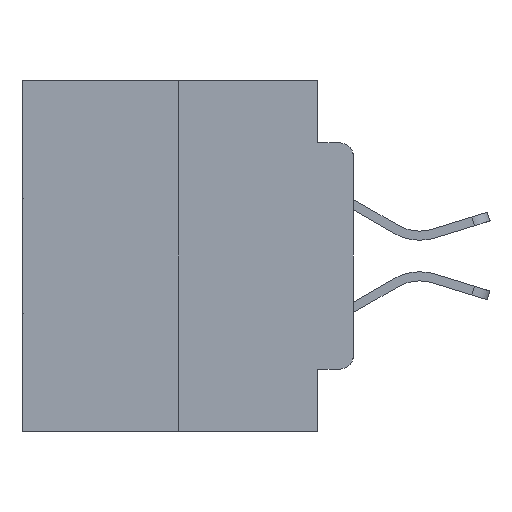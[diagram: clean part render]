
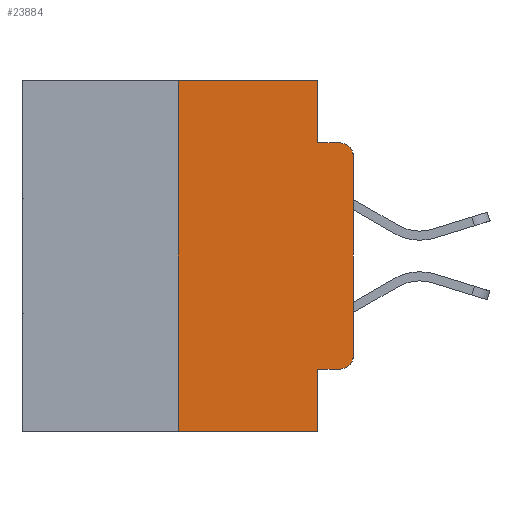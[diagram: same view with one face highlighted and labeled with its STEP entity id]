
A CAD part, left-side view. The second image highlights one B-rep face of the part: STEP entity #23884.
In plain terms, the highlighted planar face has unit normal (-1, 0, 0).
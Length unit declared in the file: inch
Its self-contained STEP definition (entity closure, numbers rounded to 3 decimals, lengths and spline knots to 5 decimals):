
#173 = CARTESIAN_POINT ( 'NONE',  ( 0., 0.051, -0.4115 ) ) ;
#317 = AXIS2_PLACEMENT_3D ( 'NONE', #12947, #27071, #15091 ) ;
#644 = CARTESIAN_POINT ( 'NONE',  ( 0., 0.051, 0. ) ) ;
#1097 = ORIENTED_EDGE ( 'NONE', *, *, #15920, .T. ) ;
#1179 = CARTESIAN_POINT ( 'NONE',  ( 0., 0.051, -0.0885 ) ) ;
#1443 = CARTESIAN_POINT ( 'NONE',  ( 0., 0., -0.1085 ) ) ;
#1916 = CARTESIAN_POINT ( 'NONE',  ( 0., 0., -0.3915 ) ) ;
#1993 = VERTEX_POINT ( 'NONE', #1443 ) ;
#2488 = DIRECTION ( 'NONE',  ( 0., -1., 0. ) ) ;
#2595 = EDGE_CURVE ( 'NONE', #9877, #24807, #21165, .T. ) ;
#2818 = DIRECTION ( 'NONE',  ( 0., 0., -1. ) ) ;
#2937 = LINE ( 'NONE', #7211, #19235 ) ;
#3059 = CARTESIAN_POINT ( 'NONE',  ( 0., 0.02, -0.0885 ) ) ;
#3100 = VERTEX_POINT ( 'NONE', #1916 ) ;
#3442 = VERTEX_POINT ( 'NONE', #3059 ) ;
#3633 = VECTOR ( 'NONE', #2488, 39.37008 ) ;
#3648 = VECTOR ( 'NONE', #11459, 39.37008 ) ;
#3704 = CARTESIAN_POINT ( 'NONE',  ( 0., 0.473, 0. ) ) ;
#4008 = VECTOR ( 'NONE', #14145, 39.37008 ) ;
#4158 = LINE ( 'NONE', #644, #20317 ) ;
#4244 = DIRECTION ( 'NONE',  ( -1., 0., 0. ) ) ;
#4581 = EDGE_CURVE ( 'NONE', #20087, #14172, #20467, .T. ) ;
#4677 = LINE ( 'NONE', #1179, #4008 ) ;
#4738 = CARTESIAN_POINT ( 'NONE',  ( 0., 0.473, -0.5 ) ) ;
#4859 = PLANE ( 'NONE',  #17080 ) ;
#5553 = AXIS2_PLACEMENT_3D ( 'NONE', #17026, #4244, #19056 ) ;
#6284 = CARTESIAN_POINT ( 'NONE',  ( 0., 0.25, -0.5 ) ) ;
#6431 = VERTEX_POINT ( 'NONE', #14095 ) ;
#6783 = DIRECTION ( 'NONE',  ( 0., -1., 0. ) ) ;
#6820 = DIRECTION ( 'NONE',  ( 0., -1., 0. ) ) ;
#7211 = CARTESIAN_POINT ( 'NONE',  ( 0., 0.051, 0. ) ) ;
#7623 = ORIENTED_EDGE ( 'NONE', *, *, #11682, .F. ) ;
#8434 = VECTOR ( 'NONE', #8769, 39.37008 ) ;
#8769 = DIRECTION ( 'NONE',  ( 0., 0., 1. ) ) ;
#8793 = VERTEX_POINT ( 'NONE', #17777 ) ;
#8986 = ORIENTED_EDGE ( 'NONE', *, *, #10101, .T. ) ;
#9210 = DIRECTION ( 'NONE',  ( 1., 0., 0. ) ) ;
#9493 = VECTOR ( 'NONE', #6820, 39.37008 ) ;
#9877 = VERTEX_POINT ( 'NONE', #26623 ) ;
#10101 = EDGE_CURVE ( 'NONE', #6431, #11656, #15154, .T. ) ;
#10368 = ORIENTED_EDGE ( 'NONE', *, *, #17141, .T. ) ;
#10548 = ORIENTED_EDGE ( 'NONE', *, *, #11519, .F. ) ;
#11210 = CIRCLE ( 'NONE', #5553, 0.02 ) ;
#11313 = EDGE_CURVE ( 'NONE', #3100, #1993, #24207, .T. ) ;
#11366 = CARTESIAN_POINT ( 'NONE',  ( 0., 0.25, 0. ) ) ;
#11459 = DIRECTION ( 'NONE',  ( 0., 0., 1. ) ) ;
#11519 = EDGE_CURVE ( 'NONE', #6431, #14172, #2937, .T. ) ;
#11656 = VERTEX_POINT ( 'NONE', #16251 ) ;
#11682 = EDGE_CURVE ( 'NONE', #8793, #3442, #4677, .T. ) ;
#11991 = ORIENTED_EDGE ( 'NONE', *, *, #2595, .F. ) ;
#12947 = CARTESIAN_POINT ( 'NONE',  ( 0., 0.02, -0.1085 ) ) ;
#14095 = CARTESIAN_POINT ( 'NONE',  ( 0., 0.051, -0.4115 ) ) ;
#14145 = DIRECTION ( 'NONE',  ( 0., -1., 0. ) ) ;
#14172 = VERTEX_POINT ( 'NONE', #18954 ) ;
#15058 = LINE ( 'NONE', #11366, #3648 ) ;
#15091 = DIRECTION ( 'NONE',  ( 0., 0., -1. ) ) ;
#15154 = LINE ( 'NONE', #173, #9493 ) ;
#15484 = EDGE_LOOP ( 'NONE', ( #18832, #1097, #7623, #16925, #11991, #20281, #16147, #10548, #8986, #10368 ) ) ;
#15590 = CIRCLE ( 'NONE', #317, 0.02 ) ;
#15767 = DIRECTION ( 'NONE',  ( 0., 0., -1. ) ) ;
#15782 = VECTOR ( 'NONE', #6783, 39.37008 ) ;
#15920 = EDGE_CURVE ( 'NONE', #1993, #3442, #15590, .T. ) ;
#16041 = FACE_OUTER_BOUND ( 'NONE', #15484, .T. ) ;
#16147 = ORIENTED_EDGE ( 'NONE', *, *, #4581, .T. ) ;
#16251 = CARTESIAN_POINT ( 'NONE',  ( 0., 0.02, -0.4115 ) ) ;
#16796 = EDGE_CURVE ( 'NONE', #24807, #8793, #4158, .T. ) ;
#16925 = ORIENTED_EDGE ( 'NONE', *, *, #16796, .F. ) ;
#17026 = CARTESIAN_POINT ( 'NONE',  ( 0., 0.02, -0.3915 ) ) ;
#17080 = AXIS2_PLACEMENT_3D ( 'NONE', #19616, #9210, #23592 ) ;
#17141 = EDGE_CURVE ( 'NONE', #11656, #3100, #11210, .T. ) ;
#17777 = CARTESIAN_POINT ( 'NONE',  ( 0., 0.051, -0.0885 ) ) ;
#18832 = ORIENTED_EDGE ( 'NONE', *, *, #11313, .T. ) ;
#18954 = CARTESIAN_POINT ( 'NONE',  ( 0., 0.051, -0.5 ) ) ;
#19056 = DIRECTION ( 'NONE',  ( 0., 0., -1. ) ) ;
#19235 = VECTOR ( 'NONE', #2818, 39.37008 ) ;
#19616 = CARTESIAN_POINT ( 'NONE',  ( 0., 0.473, 0. ) ) ;
#20087 = VERTEX_POINT ( 'NONE', #6284 ) ;
#20281 = ORIENTED_EDGE ( 'NONE', *, *, #20363, .F. ) ;
#20317 = VECTOR ( 'NONE', #15767, 39.37008 ) ;
#20363 = EDGE_CURVE ( 'NONE', #20087, #9877, #15058, .T. ) ;
#20467 = LINE ( 'NONE', #4738, #3633 ) ;
#21165 = LINE ( 'NONE', #3704, #15782 ) ;
#23167 = CARTESIAN_POINT ( 'NONE',  ( 0., 0., 0. ) ) ;
#23592 = DIRECTION ( 'NONE',  ( 0., 0., -1. ) ) ;
#23884 = ADVANCED_FACE ( 'NONE', ( #16041 ), #4859, .F. ) ;
#24207 = LINE ( 'NONE', #23167, #8434 ) ;
#24807 = VERTEX_POINT ( 'NONE', #26580 ) ;
#26580 = CARTESIAN_POINT ( 'NONE',  ( 0., 0.051, 0. ) ) ;
#26623 = CARTESIAN_POINT ( 'NONE',  ( 0., 0.25, 0. ) ) ;
#27071 = DIRECTION ( 'NONE',  ( -1., 0., 0. ) ) ;
